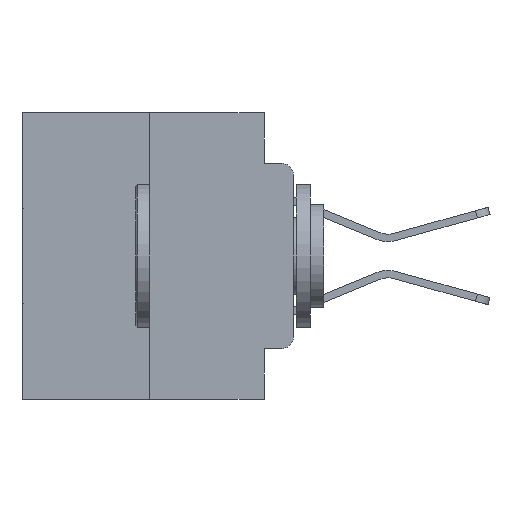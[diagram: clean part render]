
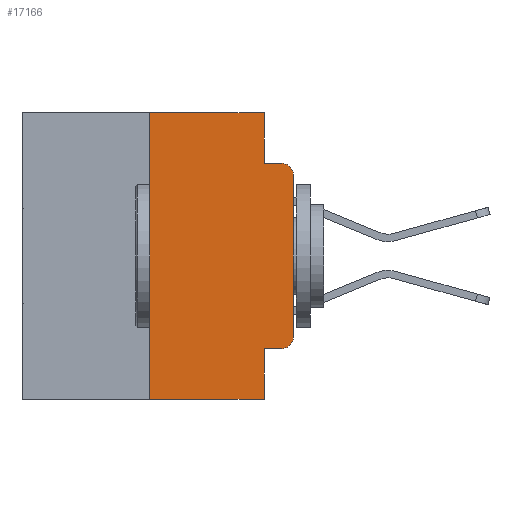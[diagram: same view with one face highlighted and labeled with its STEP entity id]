
A CAD part, left-side view. The second image highlights one B-rep face of the part: STEP entity #17166.
In plain terms, the highlighted planar face has unit normal (-1, 0, 0).
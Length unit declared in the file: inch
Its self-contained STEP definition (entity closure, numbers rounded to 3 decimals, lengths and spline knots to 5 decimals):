
#12 = DIRECTION ( 'NONE',  ( 0., 0., -1. ) ) ;
#58 = CARTESIAN_POINT ( 'NONE',  ( 0., 0.25, 0. ) ) ;
#208 = DIRECTION ( 'NONE',  ( 0., 0., -1. ) ) ;
#287 = VECTOR ( 'NONE', #12, 39.37008 ) ;
#711 = FACE_OUTER_BOUND ( 'NONE', #23533, .T. ) ;
#1627 = CIRCLE ( 'NONE', #22550, 0.02 ) ;
#1757 = VERTEX_POINT ( 'NONE', #26209 ) ;
#2243 = AXIS2_PLACEMENT_3D ( 'NONE', #29039, #5824, #28732 ) ;
#2313 = EDGE_CURVE ( 'NONE', #3858, #28855, #6311, .T. ) ;
#2336 = CARTESIAN_POINT ( 'NONE',  ( 0., 0.051, 0. ) ) ;
#2757 = VERTEX_POINT ( 'NONE', #5964 ) ;
#2840 = EDGE_CURVE ( 'NONE', #5056, #1757, #29165, .T. ) ;
#3122 = CARTESIAN_POINT ( 'NONE',  ( 0., 0.473, 0. ) ) ;
#3332 = EDGE_CURVE ( 'NONE', #16971, #18387, #3343, .T. ) ;
#3343 = LINE ( 'NONE', #3645, #9304 ) ;
#3645 = CARTESIAN_POINT ( 'NONE',  ( 0., 0.473, 0. ) ) ;
#3680 = DIRECTION ( 'NONE',  ( 0., -1., 0. ) ) ;
#3858 = VERTEX_POINT ( 'NONE', #25003 ) ;
#3952 = EDGE_CURVE ( 'NONE', #1757, #22710, #1627, .T. ) ;
#4218 = CARTESIAN_POINT ( 'NONE',  ( 0., 0.02, -0.3915 ) ) ;
#5056 = VERTEX_POINT ( 'NONE', #28803 ) ;
#5371 = ORIENTED_EDGE ( 'NONE', *, *, #3332, .F. ) ;
#5606 = CIRCLE ( 'NONE', #2243, 0.02 ) ;
#5824 = DIRECTION ( 'NONE',  ( -1., 0., 0. ) ) ;
#5833 = VECTOR ( 'NONE', #21784, 39.37008 ) ;
#5964 = CARTESIAN_POINT ( 'NONE',  ( 0., 0., -0.1085 ) ) ;
#6001 = CARTESIAN_POINT ( 'NONE',  ( 0., 0.473, -0.5 ) ) ;
#6201 = EDGE_CURVE ( 'NONE', #3858, #16971, #23085, .T. ) ;
#6237 = EDGE_CURVE ( 'NONE', #18387, #19399, #13918, .T. ) ;
#6311 = LINE ( 'NONE', #6001, #10249 ) ;
#7184 = DIRECTION ( 'NONE',  ( 0., 0., 1. ) ) ;
#7607 = ORIENTED_EDGE ( 'NONE', *, *, #2313, .T. ) ;
#8206 = DIRECTION ( 'NONE',  ( 0., -1., 0. ) ) ;
#8447 = DIRECTION ( 'NONE',  ( 0., 0., 1. ) ) ;
#8460 = CARTESIAN_POINT ( 'NONE',  ( 0., 0.051, 0. ) ) ;
#9154 = VECTOR ( 'NONE', #8447, 39.37008 ) ;
#9255 = VECTOR ( 'NONE', #3680, 39.37008 ) ;
#9304 = VECTOR ( 'NONE', #8206, 39.37008 ) ;
#9862 = VECTOR ( 'NONE', #208, 39.37008 ) ;
#10249 = VECTOR ( 'NONE', #19589, 39.37008 ) ;
#10354 = VECTOR ( 'NONE', #7184, 39.37008 ) ;
#10360 = LINE ( 'NONE', #28819, #5833 ) ;
#10824 = CARTESIAN_POINT ( 'NONE',  ( 0., 0.02, -0.0885 ) ) ;
#11069 = CARTESIAN_POINT ( 'NONE',  ( 0., 0., -0.3915 ) ) ;
#11246 = DIRECTION ( 'NONE',  ( -1., 0., 0. ) ) ;
#11952 = ORIENTED_EDGE ( 'NONE', *, *, #23306, .F. ) ;
#11968 = AXIS2_PLACEMENT_3D ( 'NONE', #3122, #15174, #12903 ) ;
#12895 = CARTESIAN_POINT ( 'NONE',  ( 0., 0., 0. ) ) ;
#12903 = DIRECTION ( 'NONE',  ( 0., 0., -1. ) ) ;
#13849 = CARTESIAN_POINT ( 'NONE',  ( 0., 0.25, 0. ) ) ;
#13918 = LINE ( 'NONE', #2336, #9862 ) ;
#14727 = CARTESIAN_POINT ( 'NONE',  ( 0., 0.051, -0.5 ) ) ;
#15174 = DIRECTION ( 'NONE',  ( 1., 0., 0. ) ) ;
#15405 = ORIENTED_EDGE ( 'NONE', *, *, #6201, .F. ) ;
#16608 = EDGE_CURVE ( 'NONE', #5056, #28855, #23335, .T. ) ;
#16971 = VERTEX_POINT ( 'NONE', #13849 ) ;
#17166 = ADVANCED_FACE ( 'NONE', ( #711 ), #28614, .F. ) ;
#17557 = CARTESIAN_POINT ( 'NONE',  ( 0., 0.051, -0.4115 ) ) ;
#18271 = ORIENTED_EDGE ( 'NONE', *, *, #3952, .T. ) ;
#18387 = VERTEX_POINT ( 'NONE', #8460 ) ;
#18671 = EDGE_CURVE ( 'NONE', #2757, #26598, #5606, .T. ) ;
#19399 = VERTEX_POINT ( 'NONE', #26335 ) ;
#19589 = DIRECTION ( 'NONE',  ( 0., -1., 0. ) ) ;
#20555 = DIRECTION ( 'NONE',  ( 0., 0., -1. ) ) ;
#20865 = ORIENTED_EDGE ( 'NONE', *, *, #27672, .T. ) ;
#21375 = ORIENTED_EDGE ( 'NONE', *, *, #2840, .T. ) ;
#21784 = DIRECTION ( 'NONE',  ( 0., -1., 0. ) ) ;
#22532 = ORIENTED_EDGE ( 'NONE', *, *, #6237, .F. ) ;
#22550 = AXIS2_PLACEMENT_3D ( 'NONE', #4218, #11246, #20555 ) ;
#22710 = VERTEX_POINT ( 'NONE', #11069 ) ;
#23085 = LINE ( 'NONE', #58, #10354 ) ;
#23306 = EDGE_CURVE ( 'NONE', #19399, #26598, #10360, .T. ) ;
#23335 = LINE ( 'NONE', #28497, #287 ) ;
#23533 = EDGE_LOOP ( 'NONE', ( #20865, #26514, #11952, #22532, #5371, #15405, #7607, #27637, #21375, #18271 ) ) ;
#24818 = LINE ( 'NONE', #12895, #9154 ) ;
#25003 = CARTESIAN_POINT ( 'NONE',  ( 0., 0.25, -0.5 ) ) ;
#26209 = CARTESIAN_POINT ( 'NONE',  ( 0., 0.02, -0.4115 ) ) ;
#26335 = CARTESIAN_POINT ( 'NONE',  ( 0., 0.051, -0.0885 ) ) ;
#26514 = ORIENTED_EDGE ( 'NONE', *, *, #18671, .T. ) ;
#26598 = VERTEX_POINT ( 'NONE', #10824 ) ;
#27637 = ORIENTED_EDGE ( 'NONE', *, *, #16608, .F. ) ;
#27672 = EDGE_CURVE ( 'NONE', #22710, #2757, #24818, .T. ) ;
#28497 = CARTESIAN_POINT ( 'NONE',  ( 0., 0.051, 0. ) ) ;
#28614 = PLANE ( 'NONE',  #11968 ) ;
#28732 = DIRECTION ( 'NONE',  ( 0., 0., -1. ) ) ;
#28803 = CARTESIAN_POINT ( 'NONE',  ( 0., 0.051, -0.4115 ) ) ;
#28819 = CARTESIAN_POINT ( 'NONE',  ( 0., 0.051, -0.0885 ) ) ;
#28855 = VERTEX_POINT ( 'NONE', #14727 ) ;
#29039 = CARTESIAN_POINT ( 'NONE',  ( 0., 0.02, -0.1085 ) ) ;
#29165 = LINE ( 'NONE', #17557, #9255 ) ;
